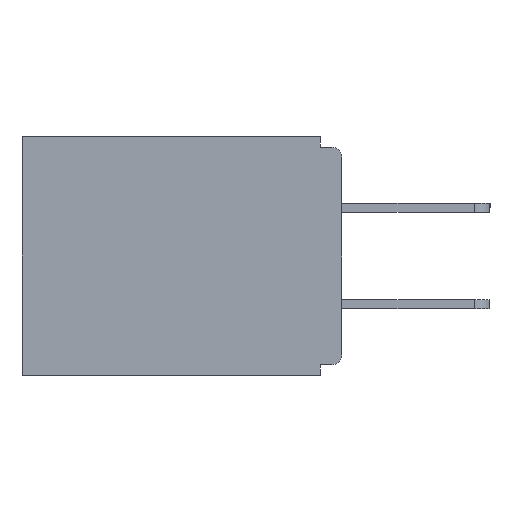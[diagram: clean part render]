
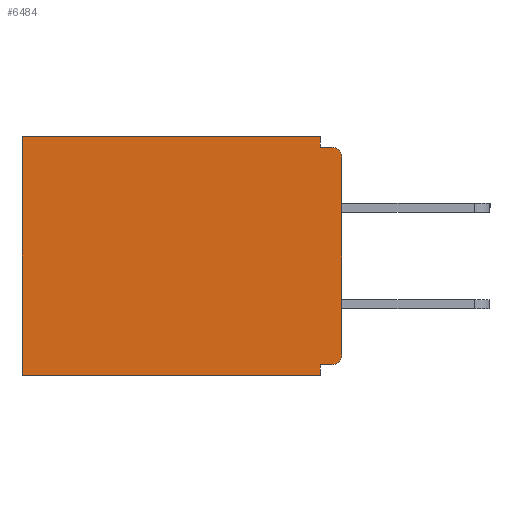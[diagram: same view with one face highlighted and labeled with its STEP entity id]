
A CAD part, left-side view. The second image highlights one B-rep face of the part: STEP entity #6484.
In plain terms, the highlighted planar face has unit normal (-1, 0, 0).
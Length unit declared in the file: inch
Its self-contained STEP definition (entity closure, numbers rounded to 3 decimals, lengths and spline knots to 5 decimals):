
#244 = ORIENTED_EDGE ( 'NONE', *, *, #16884, .T. ) ;
#376 = DIRECTION ( 'NONE',  ( 0., 0., -1. ) ) ;
#796 = LINE ( 'NONE', #4607, #3281 ) ;
#812 = VECTOR ( 'NONE', #13088, 39.37008 ) ;
#1519 = LINE ( 'NONE', #21624, #6477 ) ;
#1556 = LINE ( 'NONE', #20860, #2778 ) ;
#2778 = VECTOR ( 'NONE', #22870, 39.37008 ) ;
#2894 = CARTESIAN_POINT ( 'NONE',  ( 0.298, 0.031, -0.328 ) ) ;
#2970 = CARTESIAN_POINT ( 'NONE',  ( 0.298, 0.46, 0. ) ) ;
#2986 = EDGE_CURVE ( 'NONE', #12622, #25695, #20448, .T. ) ;
#3221 = VERTEX_POINT ( 'NONE', #16699 ) ;
#3281 = VECTOR ( 'NONE', #376, 39.37008 ) ;
#4028 = DIRECTION ( 'NONE',  ( 0., -1., 0. ) ) ;
#4083 = EDGE_CURVE ( 'NONE', #16637, #22254, #1519, .T. ) ;
#4202 = LINE ( 'NONE', #4626, #24208 ) ;
#4592 = VECTOR ( 'NONE', #18660, 39.37008 ) ;
#4607 = CARTESIAN_POINT ( 'NONE',  ( 0.298, 0., 0. ) ) ;
#4626 = CARTESIAN_POINT ( 'NONE',  ( 0.298, 0.46, 0. ) ) ;
#4716 = EDGE_CURVE ( 'NONE', #23200, #19167, #13055, .T. ) ;
#4969 = AXIS2_PLACEMENT_3D ( 'NONE', #17833, #18187, #10021 ) ;
#6477 = VECTOR ( 'NONE', #19445, 39.37008 ) ;
#6484 = ADVANCED_FACE ( 'NONE', ( #7310 ), #16217, .F. ) ;
#7310 = FACE_OUTER_BOUND ( 'NONE', #11769, .T. ) ;
#7731 = CARTESIAN_POINT ( 'NONE',  ( 0.298, 0.015, -0.015 ) ) ;
#8918 = DIRECTION ( 'NONE',  ( 0., 0., -1. ) ) ;
#8961 = ORIENTED_EDGE ( 'NONE', *, *, #15281, .F. ) ;
#10021 = DIRECTION ( 'NONE',  ( 0., 0., -1. ) ) ;
#10058 = CARTESIAN_POINT ( 'NONE',  ( 0.298, 0., 0. ) ) ;
#10064 = CARTESIAN_POINT ( 'NONE',  ( 0.298, 0.46, -0.343 ) ) ;
#10498 = CARTESIAN_POINT ( 'NONE',  ( 0.298, 0.031, -0.343 ) ) ;
#10543 = VECTOR ( 'NONE', #18046, 39.37008 ) ;
#11004 = DIRECTION ( 'NONE',  ( -1., 0., 0. ) ) ;
#11469 = LINE ( 'NONE', #16911, #812 ) ;
#11769 = EDGE_LOOP ( 'NONE', ( #19778, #13092, #8961, #14961, #244, #13749, #25514, #21700, #14236, #17236 ) ) ;
#12504 = CARTESIAN_POINT ( 'NONE',  ( 0.298, 0., -0.03 ) ) ;
#12622 = VERTEX_POINT ( 'NONE', #12504 ) ;
#12807 = CARTESIAN_POINT ( 'NONE',  ( 0.298, 0.015, -0.03 ) ) ;
#13009 = CARTESIAN_POINT ( 'NONE',  ( 0.298, 0.031, 0. ) ) ;
#13055 = LINE ( 'NONE', #10058, #10543 ) ;
#13088 = DIRECTION ( 'NONE',  ( 0., 0., -1. ) ) ;
#13092 = ORIENTED_EDGE ( 'NONE', *, *, #22343, .F. ) ;
#13150 = LINE ( 'NONE', #19752, #16565 ) ;
#13749 = ORIENTED_EDGE ( 'NONE', *, *, #19498, .F. ) ;
#14236 = ORIENTED_EDGE ( 'NONE', *, *, #15432, .T. ) ;
#14961 = ORIENTED_EDGE ( 'NONE', *, *, #4716, .T. ) ;
#15281 = EDGE_CURVE ( 'NONE', #23200, #3221, #17714, .T. ) ;
#15432 = EDGE_CURVE ( 'NONE', #16637, #17332, #25862, .T. ) ;
#16217 = PLANE ( 'NONE',  #4969 ) ;
#16565 = VECTOR ( 'NONE', #4028, 39.37008 ) ;
#16637 = VERTEX_POINT ( 'NONE', #21336 ) ;
#16699 = CARTESIAN_POINT ( 'NONE',  ( 0.298, 0.031, -0.015 ) ) ;
#16884 = EDGE_CURVE ( 'NONE', #19167, #19769, #4202, .T. ) ;
#16911 = CARTESIAN_POINT ( 'NONE',  ( 0.298, 0.031, -0.343 ) ) ;
#17236 = ORIENTED_EDGE ( 'NONE', *, *, #25300, .F. ) ;
#17332 = VERTEX_POINT ( 'NONE', #18492 ) ;
#17714 = LINE ( 'NONE', #10498, #4592 ) ;
#17833 = CARTESIAN_POINT ( 'NONE',  ( 0.298, 0., 0. ) ) ;
#18046 = DIRECTION ( 'NONE',  ( 0., 1., 0. ) ) ;
#18187 = DIRECTION ( 'NONE',  ( 1., 0., 0. ) ) ;
#18492 = CARTESIAN_POINT ( 'NONE',  ( 0.298, 0., -0.313 ) ) ;
#18660 = DIRECTION ( 'NONE',  ( 0., 0., -1. ) ) ;
#18916 = DIRECTION ( 'NONE',  ( 0., 0., -1. ) ) ;
#19009 = CARTESIAN_POINT ( 'NONE',  ( 0.298, 0.015, -0.313 ) ) ;
#19167 = VERTEX_POINT ( 'NONE', #2970 ) ;
#19445 = DIRECTION ( 'NONE',  ( 0., 1., 0. ) ) ;
#19498 = EDGE_CURVE ( 'NONE', #24913, #19769, #1556, .T. ) ;
#19752 = CARTESIAN_POINT ( 'NONE',  ( 0.298, 0., -0.015 ) ) ;
#19769 = VERTEX_POINT ( 'NONE', #10064 ) ;
#19778 = ORIENTED_EDGE ( 'NONE', *, *, #2986, .T. ) ;
#20448 = CIRCLE ( 'NONE', #22166, 0.015 ) ;
#20858 = DIRECTION ( 'NONE',  ( -1., 0., 0. ) ) ;
#20860 = CARTESIAN_POINT ( 'NONE',  ( 0.298, 0., -0.343 ) ) ;
#21242 = CARTESIAN_POINT ( 'NONE',  ( 0.298, 0.031, -0.343 ) ) ;
#21336 = CARTESIAN_POINT ( 'NONE',  ( 0.298, 0.015, -0.328 ) ) ;
#21624 = CARTESIAN_POINT ( 'NONE',  ( 0.298, 0., -0.328 ) ) ;
#21700 = ORIENTED_EDGE ( 'NONE', *, *, #4083, .F. ) ;
#22166 = AXIS2_PLACEMENT_3D ( 'NONE', #12807, #20858, #8918 ) ;
#22254 = VERTEX_POINT ( 'NONE', #2894 ) ;
#22343 = EDGE_CURVE ( 'NONE', #3221, #25695, #13150, .T. ) ;
#22870 = DIRECTION ( 'NONE',  ( 0., 1., 0. ) ) ;
#23200 = VERTEX_POINT ( 'NONE', #13009 ) ;
#23255 = AXIS2_PLACEMENT_3D ( 'NONE', #19009, #11004, #18916 ) ;
#24208 = VECTOR ( 'NONE', #24477, 39.37008 ) ;
#24326 = EDGE_CURVE ( 'NONE', #22254, #24913, #11469, .T. ) ;
#24477 = DIRECTION ( 'NONE',  ( 0., 0., -1. ) ) ;
#24913 = VERTEX_POINT ( 'NONE', #21242 ) ;
#25300 = EDGE_CURVE ( 'NONE', #12622, #17332, #796, .T. ) ;
#25514 = ORIENTED_EDGE ( 'NONE', *, *, #24326, .F. ) ;
#25695 = VERTEX_POINT ( 'NONE', #7731 ) ;
#25862 = CIRCLE ( 'NONE', #23255, 0.015 ) ;
